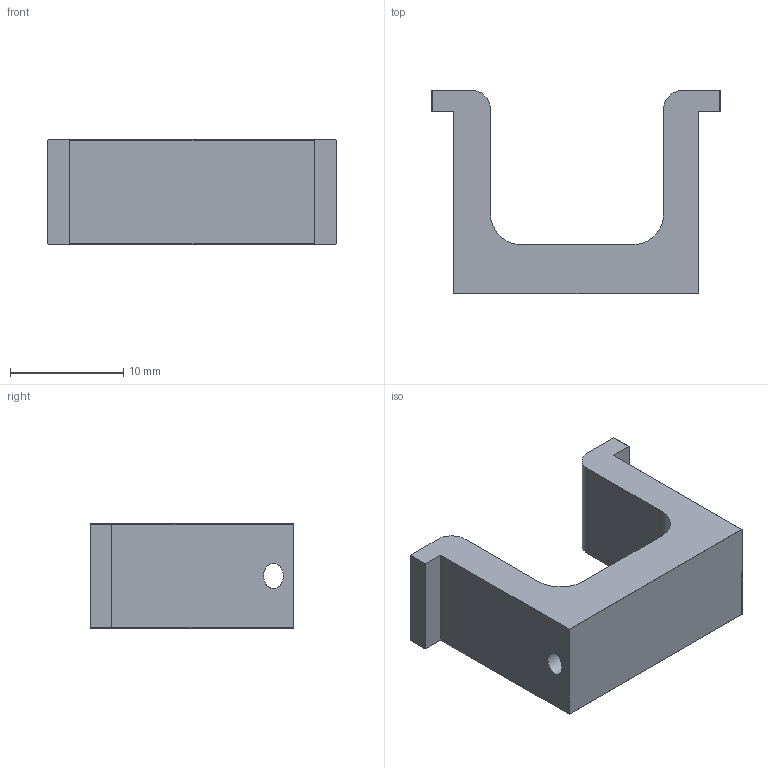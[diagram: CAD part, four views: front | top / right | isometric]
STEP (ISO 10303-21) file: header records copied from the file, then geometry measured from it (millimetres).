
FILE_DESCRIPTION(/* description */ ('STEP AP214'),/* implementation_level */ '2;1');
FILE_NAME(/* name */ 'Rear_RailPNineNineRails Release.stp',/* time_stamp */ '2022-05-10T17:49:01-05:00',/* author */ ('johne'),/* organization */ (''),/* preprocessor_version */ 'ST-DEVELOPER v18.1',/* originating_system */ 'Autodesk Inventor 2020',/* authorisation */ '');
FILE_SCHEMA (('AUTOMOTIVE_DESIGN { 1 0 10303 214 3 1 1 }'));
Length unit declared in the file: millimetre
Products named in the file (1): Rear_RailPNineNineRails (1)
Bounding box: 25.51 x 17.93 x 9.2 mm (x, y, z)
Volume: 1667.6 mm3; surface area: 1519.5 mm2
Topology: 1 solids, 1 shells, 35 faces, 89 edges, 56 vertices
Faces by surface type: plane 30, cylinder 4, bspline 1
Entity records: 1093 total; most frequent: CARTESIAN_POINT 198, ORIENTED_EDGE 178, DIRECTION 171, EDGE_CURVE 89, LINE 77, VECTOR 77, VERTEX_POINT 56, AXIS2_PLACEMENT_3D 47
